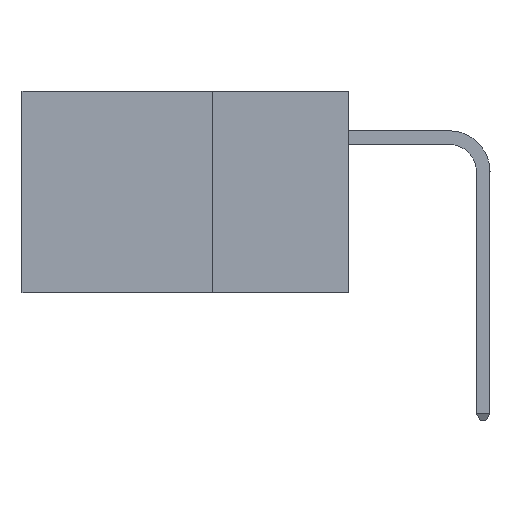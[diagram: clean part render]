
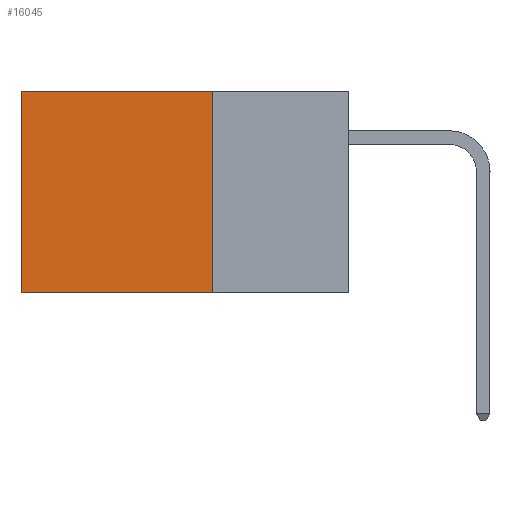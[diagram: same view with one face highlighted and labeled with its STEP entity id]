
A CAD part, left-side view. The second image highlights one B-rep face of the part: STEP entity #16045.
In plain terms, the highlighted planar face has unit normal (-1, 0, 0).
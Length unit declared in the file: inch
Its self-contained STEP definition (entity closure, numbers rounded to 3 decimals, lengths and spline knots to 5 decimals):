
#760 = EDGE_CURVE ( 'NONE', #13559, #26630, #25958, .T. ) ;
#1728 = EDGE_LOOP ( 'NONE', ( #47078, #38828, #46256, #34078 ) ) ;
#1860 = VECTOR ( 'NONE', #38740, 39.37008 ) ;
#3941 = DIRECTION ( 'NONE',  ( 0., 0., -1. ) ) ;
#5643 = VECTOR ( 'NONE', #9182, 39.37008 ) ;
#8392 = FACE_OUTER_BOUND ( 'NONE', #1728, .T. ) ;
#9182 = DIRECTION ( 'NONE',  ( 0., 1., 0. ) ) ;
#9982 = EDGE_CURVE ( 'NONE', #11323, #26630, #32400, .T. ) ;
#11323 = VERTEX_POINT ( 'NONE', #23685 ) ;
#12996 = CARTESIAN_POINT ( 'NONE',  ( 0.2875, 0.25, -0.37 ) ) ;
#13559 = VERTEX_POINT ( 'NONE', #29361 ) ;
#16045 = ADVANCED_FACE ( 'NONE', ( #8392 ), #45845, .F. ) ;
#18266 = EDGE_CURVE ( 'NONE', #29019, #11323, #24329, .T. ) ;
#22607 = LINE ( 'NONE', #40922, #39406 ) ;
#22954 = CARTESIAN_POINT ( 'NONE',  ( 0.2875, 0.25, 0. ) ) ;
#23685 = CARTESIAN_POINT ( 'NONE',  ( 0.2875, 0.6, 0. ) ) ;
#24329 = LINE ( 'NONE', #43995, #43447 ) ;
#25087 = CARTESIAN_POINT ( 'NONE',  ( 0.2875, 0.25, 0. ) ) ;
#25958 = LINE ( 'NONE', #12996, #5643 ) ;
#26630 = VERTEX_POINT ( 'NONE', #37236 ) ;
#26823 = DIRECTION ( 'NONE',  ( 1., 0., 0. ) ) ;
#29019 = VERTEX_POINT ( 'NONE', #25087 ) ;
#29361 = CARTESIAN_POINT ( 'NONE',  ( 0.2875, 0.25, -0.37 ) ) ;
#32400 = LINE ( 'NONE', #34909, #1860 ) ;
#33407 = DIRECTION ( 'NONE',  ( 0., 0., -1. ) ) ;
#33579 = AXIS2_PLACEMENT_3D ( 'NONE', #22954, #26823, #3941 ) ;
#34078 = ORIENTED_EDGE ( 'NONE', *, *, #18266, .T. ) ;
#34909 = CARTESIAN_POINT ( 'NONE',  ( 0.2875, 0.6, 0. ) ) ;
#37236 = CARTESIAN_POINT ( 'NONE',  ( 0.2875, 0.6, -0.37 ) ) ;
#38740 = DIRECTION ( 'NONE',  ( 0., 0., -1. ) ) ;
#38828 = ORIENTED_EDGE ( 'NONE', *, *, #760, .F. ) ;
#39406 = VECTOR ( 'NONE', #33407, 39.37008 ) ;
#40922 = CARTESIAN_POINT ( 'NONE',  ( 0.2875, 0.25, 0. ) ) ;
#43024 = EDGE_CURVE ( 'NONE', #29019, #13559, #22607, .T. ) ;
#43447 = VECTOR ( 'NONE', #47839, 39.37008 ) ;
#43995 = CARTESIAN_POINT ( 'NONE',  ( 0.2875, 0.25, 0. ) ) ;
#45845 = PLANE ( 'NONE',  #33579 ) ;
#46256 = ORIENTED_EDGE ( 'NONE', *, *, #43024, .F. ) ;
#47078 = ORIENTED_EDGE ( 'NONE', *, *, #9982, .T. ) ;
#47839 = DIRECTION ( 'NONE',  ( 0., 1., 0. ) ) ;
